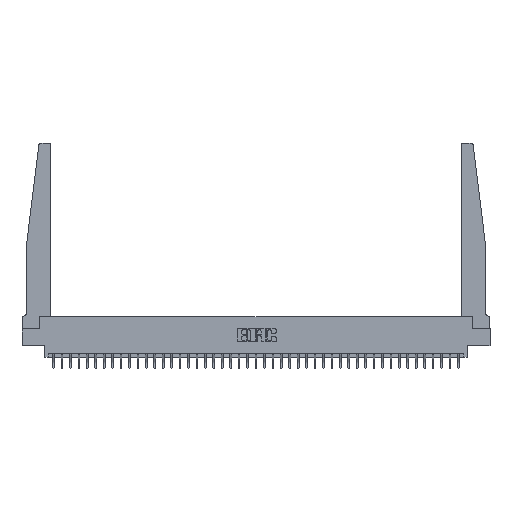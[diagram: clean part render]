
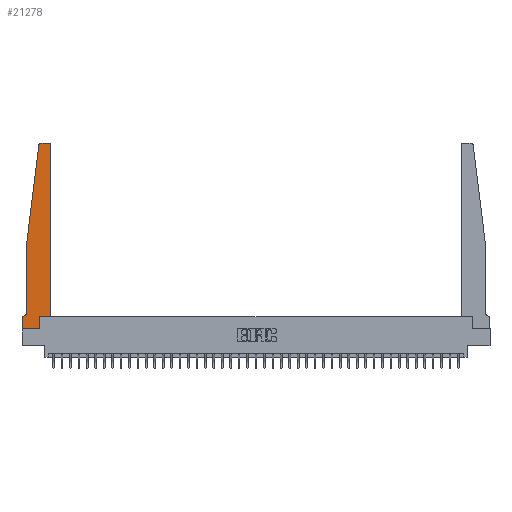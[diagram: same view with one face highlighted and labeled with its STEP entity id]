
A CAD part, top view. The second image highlights one B-rep face of the part: STEP entity #21278.
In plain terms, the highlighted planar face has unit normal (0, 0, 1).
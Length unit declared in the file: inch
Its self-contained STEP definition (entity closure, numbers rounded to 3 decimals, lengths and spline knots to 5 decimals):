
#150 = EDGE_LOOP ( 'NONE', ( #10854, #33148, #22354, #13411, #34640, #35879, #18020, #13634, #28224, #25652, #7365, #17060 ) ) ;
#209 = EDGE_CURVE ( 'NONE', #3298, #11343, #16407, .T. ) ;
#624 = DIRECTION ( 'NONE',  ( 1., 0., 0. ) ) ;
#707 = VERTEX_POINT ( 'NONE', #35987 ) ;
#1455 = EDGE_CURVE ( 'NONE', #26899, #3298, #25114, .T. ) ;
#1685 = CARTESIAN_POINT ( 'NONE',  ( 0.25, 2.75, 0.37 ) ) ;
#1793 = CARTESIAN_POINT ( 'NONE',  ( 0.27653, 2.72, 0.37 ) ) ;
#2177 = LINE ( 'NONE', #35559, #18304 ) ;
#2597 = VECTOR ( 'NONE', #20030, 39.37008 ) ;
#3124 = FACE_OUTER_BOUND ( 'NONE', #150, .T. ) ;
#3200 = CARTESIAN_POINT ( 'NONE',  ( 0., 0., 0.37 ) ) ;
#3287 = CARTESIAN_POINT ( 'NONE',  ( 0.065, 1.25, 0.37 ) ) ;
#3298 = VERTEX_POINT ( 'NONE', #31086 ) ;
#4387 = LINE ( 'NONE', #34990, #17167 ) ;
#4537 = LINE ( 'NONE', #20879, #36294 ) ;
#4801 = DIRECTION ( 'NONE',  ( 0., 1., 0. ) ) ;
#5919 = PLANE ( 'NONE',  #34901 ) ;
#5993 = CARTESIAN_POINT ( 'NONE',  ( 0.395, 2.72, 0.37 ) ) ;
#6916 = CARTESIAN_POINT ( 'NONE',  ( 0., 0.1875, 0.37 ) ) ;
#7365 = ORIENTED_EDGE ( 'NONE', *, *, #35997, .T. ) ;
#7743 = DIRECTION ( 'NONE',  ( 1., 0., 0. ) ) ;
#7772 = CARTESIAN_POINT ( 'NONE',  ( 0.2605, 0.18, 0.37 ) ) ;
#7900 = CARTESIAN_POINT ( 'NONE',  ( 0.425, 0.18, 0.37 ) ) ;
#8709 = LINE ( 'NONE', #11122, #2597 ) ;
#8973 = CIRCLE ( 'NONE', #29699, 0.03 ) ;
#9582 = CARTESIAN_POINT ( 'NONE',  ( 0.015, 0.2375, 0.37 ) ) ;
#9712 = EDGE_CURVE ( 'NONE', #11438, #24759, #19187, .T. ) ;
#10256 = CARTESIAN_POINT ( 'NONE',  ( 0.2605, 0.18, 0.37 ) ) ;
#10354 = DIRECTION ( 'NONE',  ( 0., -1., 0. ) ) ;
#10854 = ORIENTED_EDGE ( 'NONE', *, *, #22501, .T. ) ;
#11122 = CARTESIAN_POINT ( 'NONE',  ( 0., 0., 0.37 ) ) ;
#11343 = VERTEX_POINT ( 'NONE', #6916 ) ;
#11438 = VERTEX_POINT ( 'NONE', #27835 ) ;
#12535 = DIRECTION ( 'NONE',  ( -1., 0., 0. ) ) ;
#13000 = LINE ( 'NONE', #7772, #30284 ) ;
#13113 = DIRECTION ( 'NONE',  ( 0., 0., 1. ) ) ;
#13411 = ORIENTED_EDGE ( 'NONE', *, *, #18241, .T. ) ;
#13634 = ORIENTED_EDGE ( 'NONE', *, *, #28190, .T. ) ;
#15513 = CARTESIAN_POINT ( 'NONE',  ( 0.24675, 2.72367, 0.37 ) ) ;
#15665 = DIRECTION ( 'NONE',  ( 0., 0., -1. ) ) ;
#15821 = VECTOR ( 'NONE', #27342, 39.37008 ) ;
#16278 = EDGE_CURVE ( 'NONE', #22767, #23480, #13000, .T. ) ;
#16407 = LINE ( 'NONE', #24938, #15821 ) ;
#16853 = CARTESIAN_POINT ( 'NONE',  ( 0., 0.1875, 0.37 ) ) ;
#17060 = ORIENTED_EDGE ( 'NONE', *, *, #23677, .T. ) ;
#17167 = VECTOR ( 'NONE', #29619, 39.37008 ) ;
#17188 = DIRECTION ( 'NONE',  ( 0., 1., 0. ) ) ;
#17411 = DIRECTION ( 'NONE',  ( 1., 0., 0. ) ) ;
#17526 = CARTESIAN_POINT ( 'NONE',  ( 0.425, 0.18, 0.37 ) ) ;
#18020 = ORIENTED_EDGE ( 'NONE', *, *, #34511, .T. ) ;
#18241 = EDGE_CURVE ( 'NONE', #22812, #26899, #4537, .T. ) ;
#18304 = VECTOR ( 'NONE', #10354, 39.37008 ) ;
#19187 = CIRCLE ( 'NONE', #35149, 0.03 ) ;
#19795 = VECTOR ( 'NONE', #17188, 39.37008 ) ;
#19980 = CARTESIAN_POINT ( 'NONE',  ( 0.065, 0.2375, 0.37 ) ) ;
#20030 = DIRECTION ( 'NONE',  ( 1., 0., 0. ) ) ;
#20264 = DIRECTION ( 'NONE',  ( 1., 0., 0. ) ) ;
#20366 = DIRECTION ( 'NONE',  ( 0., 0., 1. ) ) ;
#20879 = CARTESIAN_POINT ( 'NONE',  ( 0.065, 1.25, 0.37 ) ) ;
#21278 = ADVANCED_FACE ( 'NONE', ( #3124 ), #5919, .T. ) ;
#21369 = EDGE_CURVE ( 'NONE', #24759, #22812, #4387, .T. ) ;
#22354 = ORIENTED_EDGE ( 'NONE', *, *, #21369, .T. ) ;
#22501 = EDGE_CURVE ( 'NONE', #707, #11438, #23972, .T. ) ;
#22687 = DIRECTION ( 'NONE',  ( 0., 0., 1. ) ) ;
#22767 = VERTEX_POINT ( 'NONE', #35554 ) ;
#22812 = VERTEX_POINT ( 'NONE', #3287 ) ;
#23480 = VERTEX_POINT ( 'NONE', #10256 ) ;
#23677 = EDGE_CURVE ( 'NONE', #32594, #707, #8973, .T. ) ;
#23972 = LINE ( 'NONE', #1685, #34950 ) ;
#24759 = VERTEX_POINT ( 'NONE', #15513 ) ;
#24938 = CARTESIAN_POINT ( 'NONE',  ( 0.065, 0.1875, 0.37 ) ) ;
#25114 = CIRCLE ( 'NONE', #29842, 0.05 ) ;
#25652 = ORIENTED_EDGE ( 'NONE', *, *, #28675, .T. ) ;
#26899 = VERTEX_POINT ( 'NONE', #19980 ) ;
#27342 = DIRECTION ( 'NONE',  ( -1., 0., 0. ) ) ;
#27835 = CARTESIAN_POINT ( 'NONE',  ( 0.27653, 2.75, 0.37 ) ) ;
#28114 = CARTESIAN_POINT ( 'NONE',  ( 0.425, 0.18, 0.37 ) ) ;
#28190 = EDGE_CURVE ( 'NONE', #33746, #22767, #8709, .T. ) ;
#28224 = ORIENTED_EDGE ( 'NONE', *, *, #16278, .T. ) ;
#28297 = LINE ( 'NONE', #28114, #19795 ) ;
#28675 = EDGE_CURVE ( 'NONE', #23480, #34992, #31621, .T. ) ;
#29399 = DIRECTION ( 'NONE',  ( 0., -1., 0. ) ) ;
#29619 = DIRECTION ( 'NONE',  ( -0.122, -0.992, 0. ) ) ;
#29699 = AXIS2_PLACEMENT_3D ( 'NONE', #5993, #22687, #20264 ) ;
#29842 = AXIS2_PLACEMENT_3D ( 'NONE', #9582, #15665, #12535 ) ;
#30284 = VECTOR ( 'NONE', #4801, 39.37008 ) ;
#31086 = CARTESIAN_POINT ( 'NONE',  ( 0.015, 0.1875, 0.37 ) ) ;
#31621 = LINE ( 'NONE', #17526, #33405 ) ;
#32594 = VERTEX_POINT ( 'NONE', #34691 ) ;
#33148 = ORIENTED_EDGE ( 'NONE', *, *, #9712, .T. ) ;
#33405 = VECTOR ( 'NONE', #624, 39.37008 ) ;
#33746 = VERTEX_POINT ( 'NONE', #3200 ) ;
#34511 = EDGE_CURVE ( 'NONE', #11343, #33746, #2177, .T. ) ;
#34640 = ORIENTED_EDGE ( 'NONE', *, *, #1455, .T. ) ;
#34691 = CARTESIAN_POINT ( 'NONE',  ( 0.425, 2.72, 0.37 ) ) ;
#34901 = AXIS2_PLACEMENT_3D ( 'NONE', #16853, #20366, #17411 ) ;
#34950 = VECTOR ( 'NONE', #35619, 39.37008 ) ;
#34990 = CARTESIAN_POINT ( 'NONE',  ( 0.065, 1.25, 0.37 ) ) ;
#34992 = VERTEX_POINT ( 'NONE', #7900 ) ;
#35149 = AXIS2_PLACEMENT_3D ( 'NONE', #1793, #13113, #7743 ) ;
#35554 = CARTESIAN_POINT ( 'NONE',  ( 0.2605, 0., 0.37 ) ) ;
#35559 = CARTESIAN_POINT ( 'NONE',  ( 0., 0., 0.37 ) ) ;
#35619 = DIRECTION ( 'NONE',  ( -1., 0., 0. ) ) ;
#35879 = ORIENTED_EDGE ( 'NONE', *, *, #209, .T. ) ;
#35987 = CARTESIAN_POINT ( 'NONE',  ( 0.395, 2.75, 0.37 ) ) ;
#35997 = EDGE_CURVE ( 'NONE', #34992, #32594, #28297, .T. ) ;
#36294 = VECTOR ( 'NONE', #29399, 39.37008 ) ;
